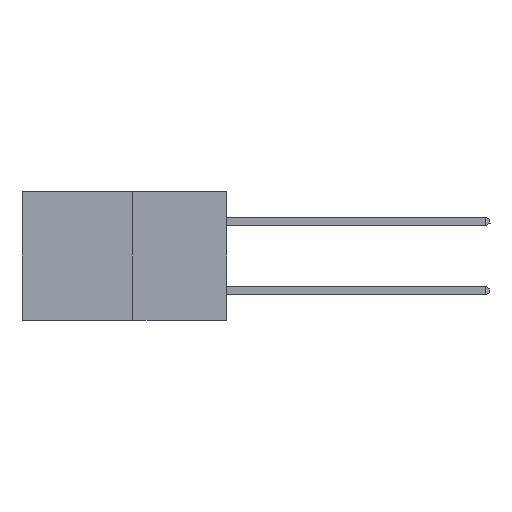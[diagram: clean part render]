
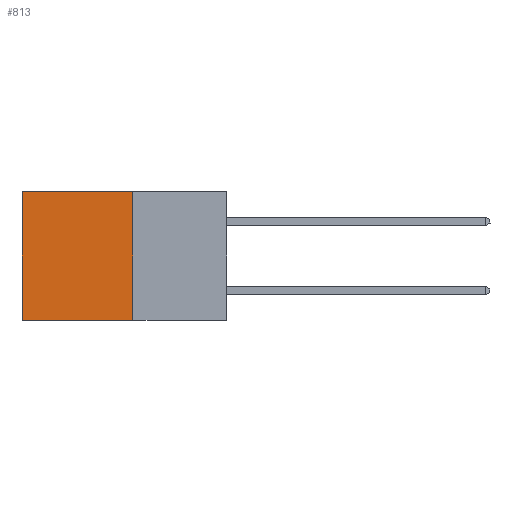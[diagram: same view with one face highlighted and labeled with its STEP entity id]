
A CAD part, left-side view. The second image highlights one B-rep face of the part: STEP entity #813.
In plain terms, the highlighted planar face has unit normal (-1, 0, 0).
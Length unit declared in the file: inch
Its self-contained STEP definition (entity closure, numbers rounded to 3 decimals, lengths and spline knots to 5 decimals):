
#118 = VECTOR ( 'NONE', #11126, 39.37008 ) ;
#747 = LINE ( 'NONE', #5436, #5275 ) ;
#813 = ADVANCED_FACE ( 'NONE', ( #6828 ), #10758, .F. ) ;
#2485 = DIRECTION ( 'NONE',  ( 0., 0., -1. ) ) ;
#2596 = ORIENTED_EDGE ( 'NONE', *, *, #8560, .T. ) ;
#2904 = LINE ( 'NONE', #6994, #118 ) ;
#3243 = ORIENTED_EDGE ( 'NONE', *, *, #4170, .F. ) ;
#3402 = ORIENTED_EDGE ( 'NONE', *, *, #8241, .T. ) ;
#3424 = EDGE_CURVE ( 'NONE', #9775, #11622, #9199, .T. ) ;
#3708 = LINE ( 'NONE', #9698, #8605 ) ;
#3934 = DIRECTION ( 'NONE',  ( 0., 0., -1. ) ) ;
#4170 = EDGE_CURVE ( 'NONE', #11622, #10748, #747, .T. ) ;
#5110 = CARTESIAN_POINT ( 'NONE',  ( 0.277, 0.59, 0. ) ) ;
#5275 = VECTOR ( 'NONE', #5746, 39.37008 ) ;
#5436 = CARTESIAN_POINT ( 'NONE',  ( 0.277, 0.27, -0.37 ) ) ;
#5728 = VERTEX_POINT ( 'NONE', #5110 ) ;
#5746 = DIRECTION ( 'NONE',  ( 0., 1., 0. ) ) ;
#6828 = FACE_OUTER_BOUND ( 'NONE', #7849, .T. ) ;
#6994 = CARTESIAN_POINT ( 'NONE',  ( 0.277, 0.27, 0. ) ) ;
#7849 = EDGE_LOOP ( 'NONE', ( #3402, #3243, #8933, #2596 ) ) ;
#8241 = EDGE_CURVE ( 'NONE', #5728, #10748, #3708, .T. ) ;
#8560 = EDGE_CURVE ( 'NONE', #9775, #5728, #2904, .T. ) ;
#8571 = DIRECTION ( 'NONE',  ( 1., 0., 0. ) ) ;
#8605 = VECTOR ( 'NONE', #2485, 39.37008 ) ;
#8782 = CARTESIAN_POINT ( 'NONE',  ( 0.277, 0.27, -0.37 ) ) ;
#8933 = ORIENTED_EDGE ( 'NONE', *, *, #3424, .F. ) ;
#9199 = LINE ( 'NONE', #8782, #11515 ) ;
#9556 = CARTESIAN_POINT ( 'NONE',  ( 0.277, 0.59, -0.37 ) ) ;
#9698 = CARTESIAN_POINT ( 'NONE',  ( 0.277, 0.59, -0.37 ) ) ;
#9775 = VERTEX_POINT ( 'NONE', #13060 ) ;
#10261 = DIRECTION ( 'NONE',  ( 0., 0., -1. ) ) ;
#10519 = CARTESIAN_POINT ( 'NONE',  ( 0.277, 0.27, -0.37 ) ) ;
#10748 = VERTEX_POINT ( 'NONE', #9556 ) ;
#10758 = PLANE ( 'NONE',  #12246 ) ;
#11126 = DIRECTION ( 'NONE',  ( 0., 1., 0. ) ) ;
#11515 = VECTOR ( 'NONE', #10261, 39.37008 ) ;
#11622 = VERTEX_POINT ( 'NONE', #10519 ) ;
#12246 = AXIS2_PLACEMENT_3D ( 'NONE', #12400, #8571, #3934 ) ;
#12400 = CARTESIAN_POINT ( 'NONE',  ( 0.277, 0.27, -0.37 ) ) ;
#13060 = CARTESIAN_POINT ( 'NONE',  ( 0.277, 0.27, 0. ) ) ;
